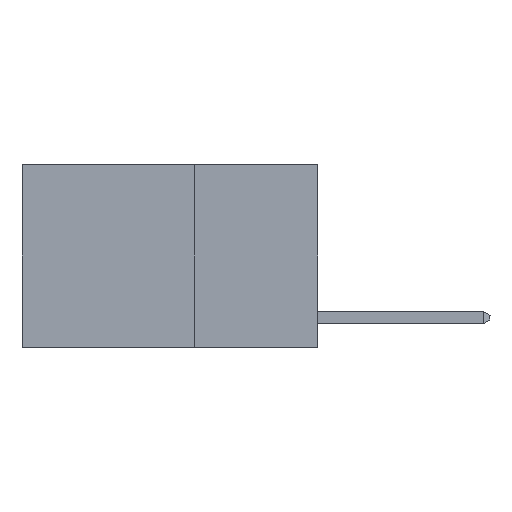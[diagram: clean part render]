
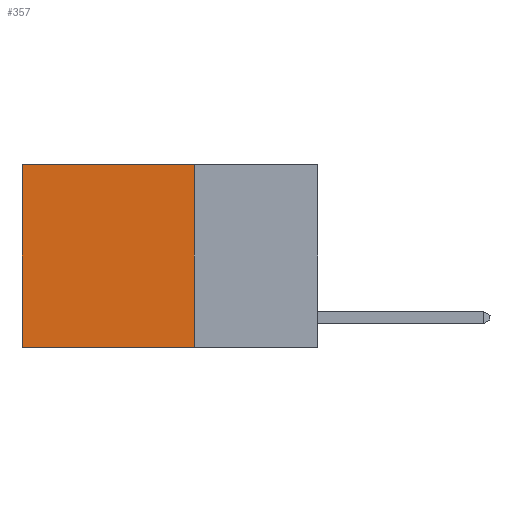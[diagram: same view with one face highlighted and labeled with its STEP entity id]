
A CAD part, left-side view. The second image highlights one B-rep face of the part: STEP entity #357.
In plain terms, the highlighted planar face has unit normal (-1, 0, 0).
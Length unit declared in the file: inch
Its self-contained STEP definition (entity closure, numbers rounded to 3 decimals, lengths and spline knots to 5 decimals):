
#357 = ADVANCED_FACE ( 'NONE', ( #6295 ), #7577, .F. ) ;
#1682 = VERTEX_POINT ( 'NONE', #7036 ) ;
#3446 = DIRECTION ( 'NONE',  ( 0., 0., -1. ) ) ;
#3829 = VECTOR ( 'NONE', #3446, 39.37008 ) ;
#4054 = DIRECTION ( 'NONE',  ( 0., 0., -1. ) ) ;
#4937 = CARTESIAN_POINT ( 'NONE',  ( 0.2625, 0.25, 0. ) ) ;
#5716 = VECTOR ( 'NONE', #11150, 39.37008 ) ;
#5765 = EDGE_CURVE ( 'NONE', #1682, #5993, #8910, .T. ) ;
#5775 = EDGE_LOOP ( 'NONE', ( #10941, #7185, #11473, #14664 ) ) ;
#5835 = DIRECTION ( 'NONE',  ( 0., 1., 0. ) ) ;
#5993 = VERTEX_POINT ( 'NONE', #6267 ) ;
#6003 = VECTOR ( 'NONE', #9163, 39.37008 ) ;
#6267 = CARTESIAN_POINT ( 'NONE',  ( 0.2625, 0.6, -0.37 ) ) ;
#6295 = FACE_OUTER_BOUND ( 'NONE', #5775, .T. ) ;
#6508 = EDGE_CURVE ( 'NONE', #15190, #5993, #7200, .T. ) ;
#6584 = VERTEX_POINT ( 'NONE', #14445 ) ;
#7036 = CARTESIAN_POINT ( 'NONE',  ( 0.2625, 0.25, -0.37 ) ) ;
#7079 = CARTESIAN_POINT ( 'NONE',  ( 0.2625, 0.25, -0.37 ) ) ;
#7185 = ORIENTED_EDGE ( 'NONE', *, *, #5765, .F. ) ;
#7194 = CARTESIAN_POINT ( 'NONE',  ( 0.2625, 0.6, 0. ) ) ;
#7200 = LINE ( 'NONE', #8430, #3829 ) ;
#7498 = EDGE_CURVE ( 'NONE', #6584, #15190, #8852, .T. ) ;
#7577 = PLANE ( 'NONE',  #9771 ) ;
#7940 = CARTESIAN_POINT ( 'NONE',  ( 0.2625, 0.25, 0. ) ) ;
#8430 = CARTESIAN_POINT ( 'NONE',  ( 0.2625, 0.6, 0. ) ) ;
#8852 = LINE ( 'NONE', #7940, #6003 ) ;
#8910 = LINE ( 'NONE', #7079, #11702 ) ;
#9163 = DIRECTION ( 'NONE',  ( 0., 1., 0. ) ) ;
#9771 = AXIS2_PLACEMENT_3D ( 'NONE', #4937, #11549, #4054 ) ;
#10846 = EDGE_CURVE ( 'NONE', #6584, #1682, #15554, .T. ) ;
#10941 = ORIENTED_EDGE ( 'NONE', *, *, #6508, .T. ) ;
#11150 = DIRECTION ( 'NONE',  ( 0., 0., -1. ) ) ;
#11473 = ORIENTED_EDGE ( 'NONE', *, *, #10846, .F. ) ;
#11549 = DIRECTION ( 'NONE',  ( 1., 0., 0. ) ) ;
#11702 = VECTOR ( 'NONE', #5835, 39.37008 ) ;
#14445 = CARTESIAN_POINT ( 'NONE',  ( 0.2625, 0.25, 0. ) ) ;
#14664 = ORIENTED_EDGE ( 'NONE', *, *, #7498, .T. ) ;
#15190 = VERTEX_POINT ( 'NONE', #7194 ) ;
#15554 = LINE ( 'NONE', #15720, #5716 ) ;
#15720 = CARTESIAN_POINT ( 'NONE',  ( 0.2625, 0.25, 0. ) ) ;
